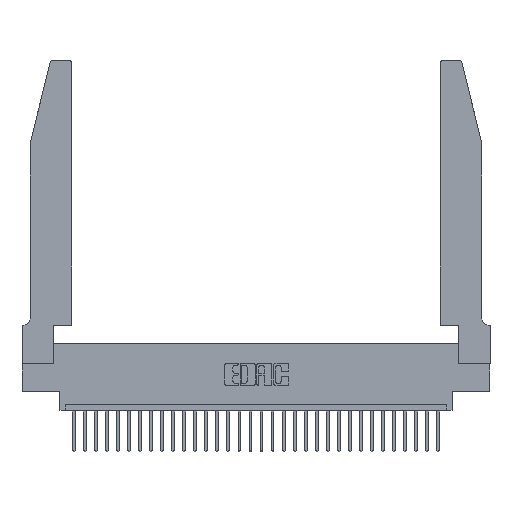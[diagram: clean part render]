
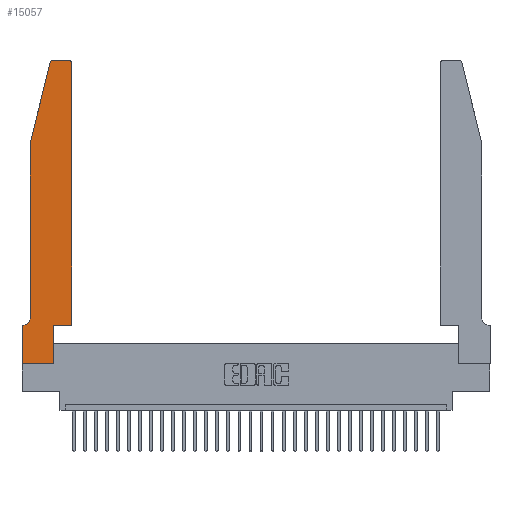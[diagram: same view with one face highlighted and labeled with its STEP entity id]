
A CAD part, top view. The second image highlights one B-rep face of the part: STEP entity #15057.
In plain terms, the highlighted planar face has unit normal (0, 0, 1).
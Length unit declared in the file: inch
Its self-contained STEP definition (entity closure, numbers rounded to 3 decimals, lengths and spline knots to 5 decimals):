
#111 = CIRCLE ( 'NONE', #25752, 0.03 ) ;
#226 = DIRECTION ( 'NONE',  ( -0.239, -0.971, 0. ) ) ;
#245 = DIRECTION ( 'NONE',  ( 1., 0., 0. ) ) ;
#779 = ORIENTED_EDGE ( 'NONE', *, *, #5589, .T. ) ;
#1146 = EDGE_CURVE ( 'NONE', #15605, #6842, #28568, .T. ) ;
#1247 = VECTOR ( 'NONE', #26321, 39.37008 ) ;
#1250 = CARTESIAN_POINT ( 'NONE',  ( 0.2865, 0.35, 0.37 ) ) ;
#1339 = DIRECTION ( 'NONE',  ( -1., 0., 0. ) ) ;
#1494 = CARTESIAN_POINT ( 'NONE',  ( 0.2865, 0.35, 0.37 ) ) ;
#1770 = CARTESIAN_POINT ( 'NONE',  ( 0., 0.35, 0.37 ) ) ;
#2306 = EDGE_CURVE ( 'NONE', #6842, #23441, #5219, .T. ) ;
#2955 = VECTOR ( 'NONE', #1339, 39.37008 ) ;
#3145 = DIRECTION ( 'NONE',  ( 0., 0., 1. ) ) ;
#3447 = VECTOR ( 'NONE', #25958, 39.37008 ) ;
#3764 = EDGE_CURVE ( 'NONE', #14847, #17472, #13894, .T. ) ;
#4113 = CARTESIAN_POINT ( 'NONE',  ( 0., 0., 0.37 ) ) ;
#4440 = DIRECTION ( 'NONE',  ( -1., 0., 0. ) ) ;
#4578 = LINE ( 'NONE', #13770, #3447 ) ;
#4991 = VECTOR ( 'NONE', #15086, 39.37008 ) ;
#5030 = EDGE_CURVE ( 'NONE', #28632, #29062, #111, .T. ) ;
#5055 = CARTESIAN_POINT ( 'NONE',  ( 0.4505, 2.72, 0.37 ) ) ;
#5219 = LINE ( 'NONE', #9296, #18156 ) ;
#5589 = EDGE_CURVE ( 'NONE', #17472, #28632, #26407, .T. ) ;
#5870 = VECTOR ( 'NONE', #226, 39.37008 ) ;
#6842 = VERTEX_POINT ( 'NONE', #18285 ) ;
#7480 = CARTESIAN_POINT ( 'NONE',  ( 0.4505, 0.35, 0.37 ) ) ;
#7822 = CARTESIAN_POINT ( 'NONE',  ( 0.284, 2.72, 0.37 ) ) ;
#9103 = AXIS2_PLACEMENT_3D ( 'NONE', #26419, #24088, #4440 ) ;
#9296 = CARTESIAN_POINT ( 'NONE',  ( 0.0755, 0.35, 0.37 ) ) ;
#9503 = CARTESIAN_POINT ( 'NONE',  ( 0., 0.35, 0.37 ) ) ;
#10086 = VECTOR ( 'NONE', #16960, 39.37008 ) ;
#10138 = ORIENTED_EDGE ( 'NONE', *, *, #20098, .T. ) ;
#10827 = CARTESIAN_POINT ( 'NONE',  ( 0.0755, 0.42, 0.37 ) ) ;
#11210 = VERTEX_POINT ( 'NONE', #11302 ) ;
#11282 = AXIS2_PLACEMENT_3D ( 'NONE', #7822, #3145, #22235 ) ;
#11302 = CARTESIAN_POINT ( 'NONE',  ( 0.25487, 2.72718, 0.37 ) ) ;
#11523 = LINE ( 'NONE', #1494, #23759 ) ;
#11635 = CARTESIAN_POINT ( 'NONE',  ( 0.284, 2.75, 0.37 ) ) ;
#11848 = ORIENTED_EDGE ( 'NONE', *, *, #24133, .T. ) ;
#11889 = CIRCLE ( 'NONE', #11282, 0.03 ) ;
#12783 = DIRECTION ( 'NONE',  ( 0., 0., 1. ) ) ;
#13119 = CARTESIAN_POINT ( 'NONE',  ( 0.4205, 2.72, 0.37 ) ) ;
#13195 = VERTEX_POINT ( 'NONE', #17915 ) ;
#13220 = DIRECTION ( 'NONE',  ( 1., 0., 0. ) ) ;
#13770 = CARTESIAN_POINT ( 'NONE',  ( 0.0755, 2., 0.37 ) ) ;
#13894 = LINE ( 'NONE', #7480, #10086 ) ;
#14017 = EDGE_CURVE ( 'NONE', #28990, #16950, #18340, .T. ) ;
#14136 = DIRECTION ( 'NONE',  ( 0., -1., 0. ) ) ;
#14190 = CARTESIAN_POINT ( 'NONE',  ( 0.2865, 0., 0.37 ) ) ;
#14778 = CARTESIAN_POINT ( 'NONE',  ( 0.0755, 2., 0.37 ) ) ;
#14831 = ORIENTED_EDGE ( 'NONE', *, *, #1146, .T. ) ;
#14847 = VERTEX_POINT ( 'NONE', #1250 ) ;
#15044 = ORIENTED_EDGE ( 'NONE', *, *, #5030, .T. ) ;
#15057 = ADVANCED_FACE ( 'NONE', ( #19441 ), #21663, .T. ) ;
#15086 = DIRECTION ( 'NONE',  ( 0., 1., 0. ) ) ;
#15480 = LINE ( 'NONE', #16882, #27723 ) ;
#15605 = VERTEX_POINT ( 'NONE', #10827 ) ;
#15790 = CARTESIAN_POINT ( 'NONE',  ( 0., 0., 0.37 ) ) ;
#16173 = CARTESIAN_POINT ( 'NONE',  ( 0.4505, 0.35, 0.37 ) ) ;
#16882 = CARTESIAN_POINT ( 'NONE',  ( 0., 0., 0.37 ) ) ;
#16950 = VERTEX_POINT ( 'NONE', #14190 ) ;
#16960 = DIRECTION ( 'NONE',  ( 1., 0., 0. ) ) ;
#17472 = VERTEX_POINT ( 'NONE', #16173 ) ;
#17915 = CARTESIAN_POINT ( 'NONE',  ( 0.0755, 2., 0.37 ) ) ;
#18156 = VECTOR ( 'NONE', #26580, 39.37008 ) ;
#18285 = CARTESIAN_POINT ( 'NONE',  ( 0.0055, 0.35, 0.37 ) ) ;
#18340 = LINE ( 'NONE', #4113, #1247 ) ;
#18664 = EDGE_CURVE ( 'NONE', #23441, #28990, #15480, .T. ) ;
#18977 = ORIENTED_EDGE ( 'NONE', *, *, #2306, .T. ) ;
#19210 = ORIENTED_EDGE ( 'NONE', *, *, #28773, .T. ) ;
#19441 = FACE_OUTER_BOUND ( 'NONE', #21274, .T. ) ;
#20098 = EDGE_CURVE ( 'NONE', #11210, #13195, #24589, .T. ) ;
#21071 = DIRECTION ( 'NONE',  ( 0., 1., 0. ) ) ;
#21245 = AXIS2_PLACEMENT_3D ( 'NONE', #9503, #12783, #245 ) ;
#21274 = EDGE_LOOP ( 'NONE', ( #31457, #19210, #10138, #11848, #14831, #18977, #29922, #23381, #30241, #27341, #779, #15044 ) ) ;
#21663 = PLANE ( 'NONE',  #21245 ) ;
#22235 = DIRECTION ( 'NONE',  ( 1., 0., 0. ) ) ;
#23171 = CARTESIAN_POINT ( 'NONE',  ( 0.2605, 2.75, 0.37 ) ) ;
#23381 = ORIENTED_EDGE ( 'NONE', *, *, #14017, .T. ) ;
#23441 = VERTEX_POINT ( 'NONE', #1770 ) ;
#23759 = VECTOR ( 'NONE', #21071, 39.37008 ) ;
#23961 = LINE ( 'NONE', #23171, #2955 ) ;
#24088 = DIRECTION ( 'NONE',  ( 0., 0., -1. ) ) ;
#24133 = EDGE_CURVE ( 'NONE', #13195, #15605, #4578, .T. ) ;
#24274 = VERTEX_POINT ( 'NONE', #11635 ) ;
#24589 = LINE ( 'NONE', #14778, #5870 ) ;
#25433 = DIRECTION ( 'NONE',  ( 0., 0., 1. ) ) ;
#25752 = AXIS2_PLACEMENT_3D ( 'NONE', #13119, #25433, #13220 ) ;
#25958 = DIRECTION ( 'NONE',  ( 0., -1., 0. ) ) ;
#26187 = CARTESIAN_POINT ( 'NONE',  ( 0.4205, 2.75, 0.37 ) ) ;
#26321 = DIRECTION ( 'NONE',  ( 1., 0., 0. ) ) ;
#26407 = LINE ( 'NONE', #30061, #4991 ) ;
#26419 = CARTESIAN_POINT ( 'NONE',  ( 0.0055, 0.42, 0.37 ) ) ;
#26580 = DIRECTION ( 'NONE',  ( -1., 0., 0. ) ) ;
#27341 = ORIENTED_EDGE ( 'NONE', *, *, #3764, .T. ) ;
#27723 = VECTOR ( 'NONE', #14136, 39.37008 ) ;
#28474 = EDGE_CURVE ( 'NONE', #16950, #14847, #11523, .T. ) ;
#28568 = CIRCLE ( 'NONE', #9103, 0.07 ) ;
#28632 = VERTEX_POINT ( 'NONE', #5055 ) ;
#28773 = EDGE_CURVE ( 'NONE', #24274, #11210, #11889, .T. ) ;
#28990 = VERTEX_POINT ( 'NONE', #15790 ) ;
#29062 = VERTEX_POINT ( 'NONE', #26187 ) ;
#29922 = ORIENTED_EDGE ( 'NONE', *, *, #18664, .T. ) ;
#30061 = CARTESIAN_POINT ( 'NONE',  ( 0.4505, 0.35, 0.37 ) ) ;
#30241 = ORIENTED_EDGE ( 'NONE', *, *, #28474, .T. ) ;
#31457 = ORIENTED_EDGE ( 'NONE', *, *, #31532, .T. ) ;
#31532 = EDGE_CURVE ( 'NONE', #29062, #24274, #23961, .T. ) ;
